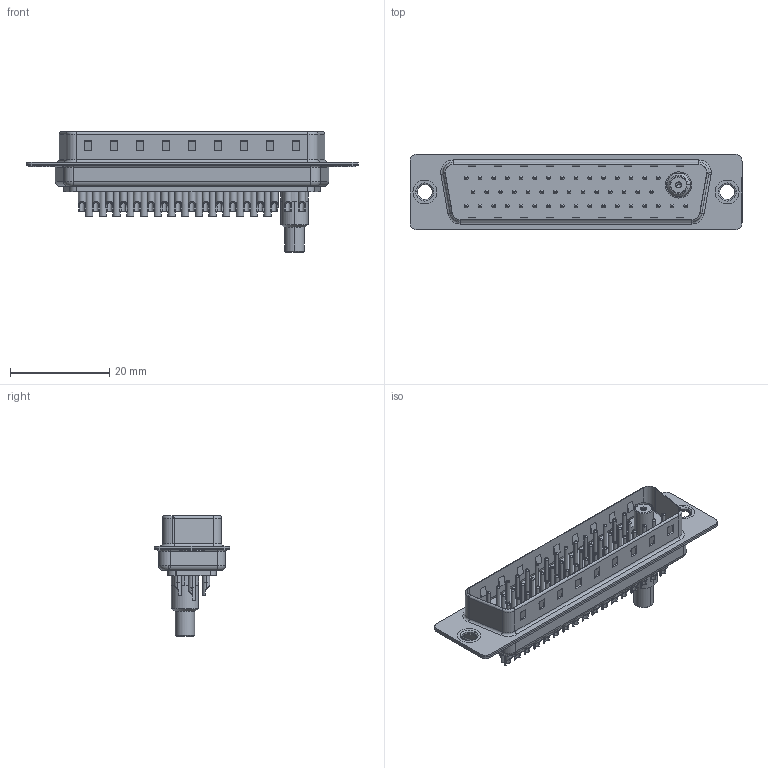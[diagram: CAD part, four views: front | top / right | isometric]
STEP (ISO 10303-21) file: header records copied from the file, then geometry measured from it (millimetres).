
FILE_DESCRIPTION (( 'STEP AP203' ), '1' );
FILE_NAME ('627-47W1622-7T1.STEP', '2019-06-20T16:45:03', ( '' ), ( '' ), 'SwSTEP 2.0', 'SolidWorks 2016', '' );
FILE_SCHEMA (( 'CONFIG_CONTROL_DESIGN' ));
Length unit declared in the file: millimetre
Products named in the file (15): 627Combo Shell Rear_50 Contacts; Co-Ax Jack Assy_SC; Insulator Socket 2; 627Combo Contact Row 1_22; 627Combo Shell Front_50 Contacts; 627Combo Contact Row 3_22; Co-Ax Jack_Solder Cup Tail; Socket_Solder Cup; 627-47W1622-7T1; Solder Cover; 627Combo Housing_47W1; Insulator Socket; 627Combo Thru Hole Rivet; 627Combo Contact Row 2_22L; Locking Collar
Assembly tree (58 placements, depth 3):
  627-47W1622-7T1
    627Combo Housing_47W1
    627Combo Shell Rear_50 Contacts
    627Combo Shell Front_50 Contacts
    627Combo Thru Hole Rivet  x2
    Co-Ax Jack Assy_SC
      Co-Ax Jack_Solder Cup Tail
      Insulator Socket
      Insulator Socket 2
      Locking Collar
      Socket_Solder Cup
      Solder Cover
    627Combo Contact Row 1_22  x15
    627Combo Contact Row 2_22L  x14
    627Combo Contact Row 3_22  x17
Bounding box: 67 x 15.3 x 24.3 mm (x, y, z)
Volume: 4671.2 mm3; surface area: 11898 mm2
Topology: 57 solids, 57 shells, 2218 faces, 5128 edges, 3132 vertices
Faces by surface type: cylinder 925, plane 657, torus 522, cone 112, bspline 2
Entity records: 31032 total; most frequent: DIRECTION 5306, CARTESIAN_POINT 4980, ORIENTED_EDGE 4476, EDGE_CURVE 2238, AXIS2_PLACEMENT_3D 2116, VERTEX_POINT 1431, EDGE_LOOP 1223, CIRCLE 1105
